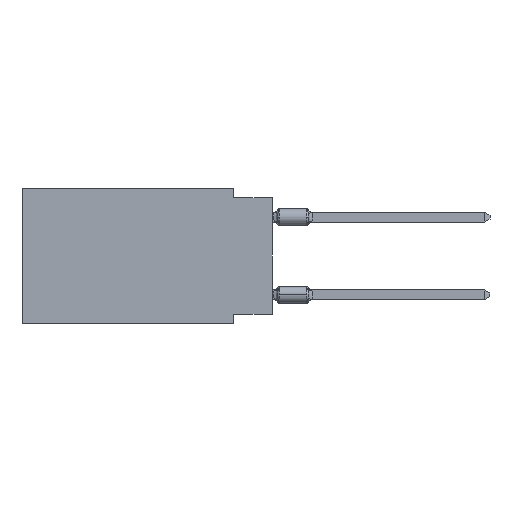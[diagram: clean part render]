
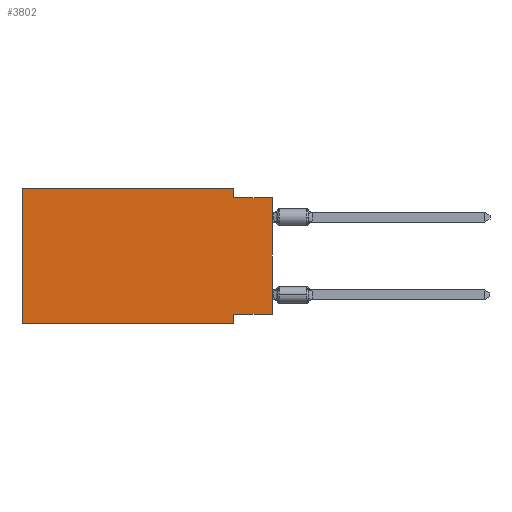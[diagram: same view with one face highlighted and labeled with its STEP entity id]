
A CAD part, left-side view. The second image highlights one B-rep face of the part: STEP entity #3802.
In plain terms, the highlighted planar face has unit normal (-1, 0, 0).
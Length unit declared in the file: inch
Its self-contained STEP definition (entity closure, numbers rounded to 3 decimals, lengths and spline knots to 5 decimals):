
#44 = CARTESIAN_POINT ( 'NONE',  ( 0., 0.1, 0. ) ) ;
#95 = CARTESIAN_POINT ( 'NONE',  ( 0., 0.645, 0. ) ) ;
#736 = ORIENTED_EDGE ( 'NONE', *, *, #2210, .F. ) ;
#1240 = EDGE_LOOP ( 'NONE', ( #11518, #18515, #13141, #17486, #7756, #9493, #736, #18801 ) ) ;
#1660 = VERTEX_POINT ( 'NONE', #16996 ) ;
#1680 = VERTEX_POINT ( 'NONE', #44 ) ;
#1830 = LINE ( 'NONE', #12632, #17406 ) ;
#1975 = VERTEX_POINT ( 'NONE', #10520 ) ;
#2045 = EDGE_CURVE ( 'NONE', #19483, #7710, #1830, .T. ) ;
#2116 = DIRECTION ( 'NONE',  ( 0., 0., -1. ) ) ;
#2144 = DIRECTION ( 'NONE',  ( 0., 0., -1. ) ) ;
#2210 = EDGE_CURVE ( 'NONE', #1975, #18484, #15948, .T. ) ;
#2678 = CARTESIAN_POINT ( 'NONE',  ( 0., 0.645, -0.35 ) ) ;
#3107 = CARTESIAN_POINT ( 'NONE',  ( 0., 0.1, -0.35 ) ) ;
#3170 = EDGE_CURVE ( 'NONE', #19483, #18484, #5498, .T. ) ;
#3802 = ADVANCED_FACE ( 'NONE', ( #14200 ), #12884, .F. ) ;
#5286 = LINE ( 'NONE', #16089, #19896 ) ;
#5297 = DIRECTION ( 'NONE',  ( 1., 0., 0. ) ) ;
#5408 = VECTOR ( 'NONE', #6243, 39.37008 ) ;
#5498 = LINE ( 'NONE', #11563, #9863 ) ;
#6243 = DIRECTION ( 'NONE',  ( 0., -1., 0. ) ) ;
#6480 = EDGE_CURVE ( 'NONE', #1660, #13138, #5286, .T. ) ;
#6965 = CARTESIAN_POINT ( 'NONE',  ( 0., 0., -0.025 ) ) ;
#7710 = VERTEX_POINT ( 'NONE', #9625 ) ;
#7756 = ORIENTED_EDGE ( 'NONE', *, *, #2045, .F. ) ;
#7900 = EDGE_CURVE ( 'NONE', #1680, #7942, #9821, .T. ) ;
#7942 = VERTEX_POINT ( 'NONE', #14880 ) ;
#7975 = DIRECTION ( 'NONE',  ( 0., 0., 1. ) ) ;
#8528 = VECTOR ( 'NONE', #19001, 39.37008 ) ;
#8942 = LINE ( 'NONE', #13206, #19300 ) ;
#9052 = EDGE_CURVE ( 'NONE', #7710, #1680, #15338, .T. ) ;
#9493 = ORIENTED_EDGE ( 'NONE', *, *, #3170, .T. ) ;
#9625 = CARTESIAN_POINT ( 'NONE',  ( 0., 0.645, 0. ) ) ;
#9821 = LINE ( 'NONE', #15976, #10598 ) ;
#9863 = VECTOR ( 'NONE', #17719, 39.37008 ) ;
#10200 = LINE ( 'NONE', #12839, #8528 ) ;
#10520 = CARTESIAN_POINT ( 'NONE',  ( 0., 0.1, -0.325 ) ) ;
#10598 = VECTOR ( 'NONE', #2144, 39.37008 ) ;
#11518 = ORIENTED_EDGE ( 'NONE', *, *, #6480, .T. ) ;
#11563 = CARTESIAN_POINT ( 'NONE',  ( 0., 0.645, -0.35 ) ) ;
#12632 = CARTESIAN_POINT ( 'NONE',  ( 0., 0.645, 0. ) ) ;
#12648 = EDGE_CURVE ( 'NONE', #7942, #13138, #8942, .T. ) ;
#12839 = CARTESIAN_POINT ( 'NONE',  ( 0., 0., -0.325 ) ) ;
#12884 = PLANE ( 'NONE',  #17203 ) ;
#13138 = VERTEX_POINT ( 'NONE', #6965 ) ;
#13141 = ORIENTED_EDGE ( 'NONE', *, *, #7900, .F. ) ;
#13206 = CARTESIAN_POINT ( 'NONE',  ( 0., 0., -0.025 ) ) ;
#14200 = FACE_OUTER_BOUND ( 'NONE', #1240, .T. ) ;
#14484 = DIRECTION ( 'NONE',  ( 0., 0., 1. ) ) ;
#14495 = DIRECTION ( 'NONE',  ( 0., 0., -1. ) ) ;
#14880 = CARTESIAN_POINT ( 'NONE',  ( 0., 0.1, -0.025 ) ) ;
#15338 = LINE ( 'NONE', #95, #5408 ) ;
#15856 = CARTESIAN_POINT ( 'NONE',  ( 0., 0.1, -0.35 ) ) ;
#15948 = LINE ( 'NONE', #15856, #17747 ) ;
#15976 = CARTESIAN_POINT ( 'NONE',  ( 0., 0.1, 0. ) ) ;
#16089 = CARTESIAN_POINT ( 'NONE',  ( 0., 0., 0. ) ) ;
#16996 = CARTESIAN_POINT ( 'NONE',  ( 0., 0., -0.325 ) ) ;
#17203 = AXIS2_PLACEMENT_3D ( 'NONE', #19229, #5297, #14495 ) ;
#17406 = VECTOR ( 'NONE', #7975, 39.37008 ) ;
#17486 = ORIENTED_EDGE ( 'NONE', *, *, #9052, .F. ) ;
#17719 = DIRECTION ( 'NONE',  ( 0., -1., 0. ) ) ;
#17747 = VECTOR ( 'NONE', #2116, 39.37008 ) ;
#18484 = VERTEX_POINT ( 'NONE', #3107 ) ;
#18515 = ORIENTED_EDGE ( 'NONE', *, *, #12648, .F. ) ;
#18801 = ORIENTED_EDGE ( 'NONE', *, *, #19719, .F. ) ;
#19001 = DIRECTION ( 'NONE',  ( 0., 1., 0. ) ) ;
#19229 = CARTESIAN_POINT ( 'NONE',  ( 0., 0.645, 0. ) ) ;
#19300 = VECTOR ( 'NONE', #19659, 39.37008 ) ;
#19483 = VERTEX_POINT ( 'NONE', #2678 ) ;
#19659 = DIRECTION ( 'NONE',  ( 0., -1., 0. ) ) ;
#19719 = EDGE_CURVE ( 'NONE', #1660, #1975, #10200, .T. ) ;
#19896 = VECTOR ( 'NONE', #14484, 39.37008 ) ;
